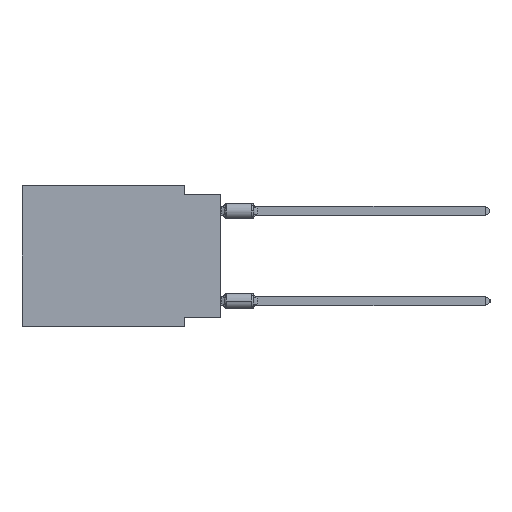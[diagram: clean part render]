
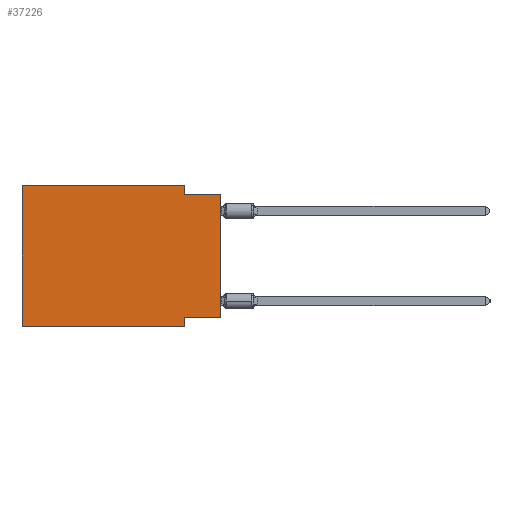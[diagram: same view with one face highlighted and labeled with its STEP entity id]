
A CAD part, left-side view. The second image highlights one B-rep face of the part: STEP entity #37226.
In plain terms, the highlighted planar face has unit normal (-1, 0, 0).
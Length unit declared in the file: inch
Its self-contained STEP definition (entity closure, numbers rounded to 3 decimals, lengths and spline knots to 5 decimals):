
#47 = VERTEX_POINT ( 'NONE', #35813 ) ;
#592 = VECTOR ( 'NONE', #20176, 39.37008 ) ;
#667 = EDGE_CURVE ( 'NONE', #14987, #12252, #11032, .T. ) ;
#1344 = EDGE_CURVE ( 'NONE', #47, #3990, #17074, .T. ) ;
#1825 = DIRECTION ( 'NONE',  ( 0., 0., 1. ) ) ;
#1854 = EDGE_CURVE ( 'NONE', #7983, #2393, #17022, .T. ) ;
#1922 = CARTESIAN_POINT ( 'NONE',  ( 0., 0.1, -0.39 ) ) ;
#2393 = VERTEX_POINT ( 'NONE', #5735 ) ;
#3990 = VERTEX_POINT ( 'NONE', #26746 ) ;
#4942 = CARTESIAN_POINT ( 'NONE',  ( 0., 0.55, -0.39 ) ) ;
#5266 = LINE ( 'NONE', #17286, #38406 ) ;
#5735 = CARTESIAN_POINT ( 'NONE',  ( 0., 0.1, -0.025 ) ) ;
#6084 = LINE ( 'NONE', #15705, #15666 ) ;
#6703 = PLANE ( 'NONE',  #10645 ) ;
#7301 = FACE_OUTER_BOUND ( 'NONE', #8528, .T. ) ;
#7318 = EDGE_CURVE ( 'NONE', #2393, #33207, #10983, .T. ) ;
#7983 = VERTEX_POINT ( 'NONE', #30966 ) ;
#8380 = CARTESIAN_POINT ( 'NONE',  ( 0., 0., -0.025 ) ) ;
#8528 = EDGE_LOOP ( 'NONE', ( #36970, #12630, #25390, #26646, #14968, #10094, #28754, #25822 ) ) ;
#9899 = DIRECTION ( 'NONE',  ( 1., 0., 0. ) ) ;
#10094 = ORIENTED_EDGE ( 'NONE', *, *, #25196, .T. ) ;
#10237 = CARTESIAN_POINT ( 'NONE',  ( 0., 0.1, -0.39 ) ) ;
#10645 = AXIS2_PLACEMENT_3D ( 'NONE', #19104, #9899, #21949 ) ;
#10738 = LINE ( 'NONE', #4942, #592 ) ;
#10983 = LINE ( 'NONE', #8380, #17599 ) ;
#11002 = DIRECTION ( 'NONE',  ( 0., 0., -1. ) ) ;
#11032 = LINE ( 'NONE', #10237, #27904 ) ;
#12252 = VERTEX_POINT ( 'NONE', #1922 ) ;
#12630 = ORIENTED_EDGE ( 'NONE', *, *, #7318, .F. ) ;
#13272 = VECTOR ( 'NONE', #1825, 39.37008 ) ;
#13652 = DIRECTION ( 'NONE',  ( 0., 0., -1. ) ) ;
#14344 = EDGE_CURVE ( 'NONE', #39497, #14987, #25790, .T. ) ;
#14574 = DIRECTION ( 'NONE',  ( 0., -1., 0. ) ) ;
#14968 = ORIENTED_EDGE ( 'NONE', *, *, #1344, .F. ) ;
#14987 = VERTEX_POINT ( 'NONE', #24319 ) ;
#15090 = DIRECTION ( 'NONE',  ( 0., 0., 1. ) ) ;
#15180 = CARTESIAN_POINT ( 'NONE',  ( 0., 0., -0.025 ) ) ;
#15666 = VECTOR ( 'NONE', #15090, 39.37008 ) ;
#15705 = CARTESIAN_POINT ( 'NONE',  ( 0., 0., 0. ) ) ;
#16146 = VECTOR ( 'NONE', #28997, 39.37008 ) ;
#16569 = VECTOR ( 'NONE', #11002, 39.37008 ) ;
#17022 = LINE ( 'NONE', #33036, #16569 ) ;
#17074 = LINE ( 'NONE', #29295, #13272 ) ;
#17286 = CARTESIAN_POINT ( 'NONE',  ( 0., 0.55, 0. ) ) ;
#17599 = VECTOR ( 'NONE', #14574, 39.37008 ) ;
#19104 = CARTESIAN_POINT ( 'NONE',  ( 0., 0.55, 0. ) ) ;
#20176 = DIRECTION ( 'NONE',  ( 0., -1., 0. ) ) ;
#21949 = DIRECTION ( 'NONE',  ( 0., 0., -1. ) ) ;
#22055 = EDGE_CURVE ( 'NONE', #39497, #33207, #6084, .T. ) ;
#23314 = DIRECTION ( 'NONE',  ( 0., -1., 0. ) ) ;
#24319 = CARTESIAN_POINT ( 'NONE',  ( 0., 0.1, -0.365 ) ) ;
#25196 = EDGE_CURVE ( 'NONE', #47, #12252, #10738, .T. ) ;
#25390 = ORIENTED_EDGE ( 'NONE', *, *, #1854, .F. ) ;
#25790 = LINE ( 'NONE', #32198, #16146 ) ;
#25822 = ORIENTED_EDGE ( 'NONE', *, *, #14344, .F. ) ;
#26438 = CARTESIAN_POINT ( 'NONE',  ( 0., 0., -0.365 ) ) ;
#26646 = ORIENTED_EDGE ( 'NONE', *, *, #28552, .F. ) ;
#26746 = CARTESIAN_POINT ( 'NONE',  ( 0., 0.55, 0. ) ) ;
#27904 = VECTOR ( 'NONE', #13652, 39.37008 ) ;
#28552 = EDGE_CURVE ( 'NONE', #3990, #7983, #5266, .T. ) ;
#28754 = ORIENTED_EDGE ( 'NONE', *, *, #667, .F. ) ;
#28997 = DIRECTION ( 'NONE',  ( 0., 1., 0. ) ) ;
#29295 = CARTESIAN_POINT ( 'NONE',  ( 0., 0.55, 0. ) ) ;
#30966 = CARTESIAN_POINT ( 'NONE',  ( 0., 0.1, 0. ) ) ;
#32198 = CARTESIAN_POINT ( 'NONE',  ( 0., 0., -0.365 ) ) ;
#33036 = CARTESIAN_POINT ( 'NONE',  ( 0., 0.1, 0. ) ) ;
#33207 = VERTEX_POINT ( 'NONE', #15180 ) ;
#35813 = CARTESIAN_POINT ( 'NONE',  ( 0., 0.55, -0.39 ) ) ;
#36970 = ORIENTED_EDGE ( 'NONE', *, *, #22055, .T. ) ;
#37226 = ADVANCED_FACE ( 'NONE', ( #7301 ), #6703, .F. ) ;
#38406 = VECTOR ( 'NONE', #23314, 39.37008 ) ;
#39497 = VERTEX_POINT ( 'NONE', #26438 ) ;
